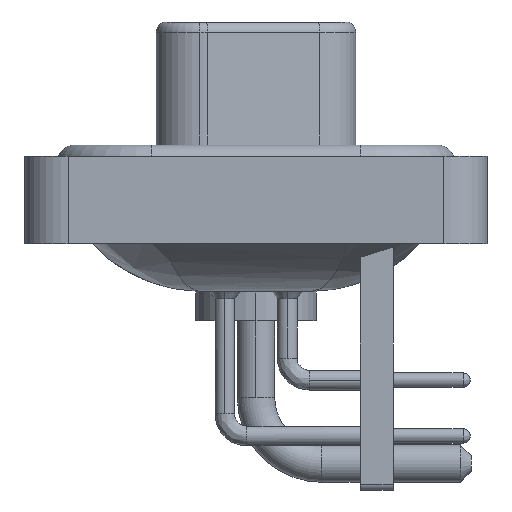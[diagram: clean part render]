
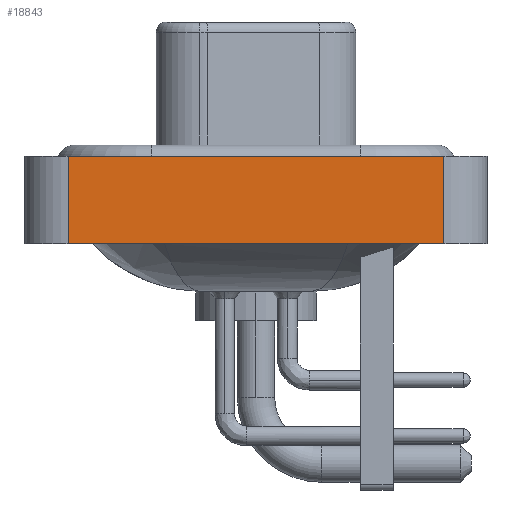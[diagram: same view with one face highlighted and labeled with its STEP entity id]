
A CAD part, left-side view. The second image highlights one B-rep face of the part: STEP entity #18843.
In plain terms, the highlighted planar face has unit normal (-1, 0, 0).
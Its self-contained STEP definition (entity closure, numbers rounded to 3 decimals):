
#630 = CARTESIAN_POINT ( 'NONE',  ( -7.25, -8.55, -3.6 ) ) ;
#1717 = EDGE_CURVE ( 'NONE', #21289, #21416, #18581, .T. ) ;
#2078 = EDGE_LOOP ( 'NONE', ( #3191, #15304, #12011, #8997 ) ) ;
#2207 = DIRECTION ( 'NONE',  ( 0., 0., 1. ) ) ;
#3191 = ORIENTED_EDGE ( 'NONE', *, *, #1717, .T. ) ;
#3697 = FACE_OUTER_BOUND ( 'NONE', #2078, .T. ) ;
#4210 = VECTOR ( 'NONE', #2207, 1000. ) ;
#4450 = DIRECTION ( 'NONE',  ( 0., -1., 0. ) ) ;
#5002 = DIRECTION ( 'NONE',  ( -1., 0., 0. ) ) ;
#5062 = LINE ( 'NONE', #12702, #16891 ) ;
#6217 = CARTESIAN_POINT ( 'NONE',  ( -7.25, -8.55, -3.6 ) ) ;
#8865 = LINE ( 'NONE', #19651, #16853 ) ;
#8997 = ORIENTED_EDGE ( 'NONE', *, *, #12492, .T. ) ;
#10084 = VERTEX_POINT ( 'NONE', #12901 ) ;
#10393 = CARTESIAN_POINT ( 'NONE',  ( -7.25, 8.55, -3.6 ) ) ;
#10760 = EDGE_CURVE ( 'NONE', #10084, #21416, #5062, .T. ) ;
#10972 = PLANE ( 'NONE',  #11722 ) ;
#11722 = AXIS2_PLACEMENT_3D ( 'NONE', #21378, #5002, #12288 ) ;
#12011 = ORIENTED_EDGE ( 'NONE', *, *, #14736, .F. ) ;
#12288 = DIRECTION ( 'NONE',  ( 0., 0., 1. ) ) ;
#12492 = EDGE_CURVE ( 'NONE', #16575, #21289, #17226, .T. ) ;
#12702 = CARTESIAN_POINT ( 'NONE',  ( -7.25, -8.55, 0.4 ) ) ;
#12901 = CARTESIAN_POINT ( 'NONE',  ( -7.25, 8.55, 0.4 ) ) ;
#14736 = EDGE_CURVE ( 'NONE', #16575, #10084, #8865, .T. ) ;
#15304 = ORIENTED_EDGE ( 'NONE', *, *, #10760, .F. ) ;
#15919 = CARTESIAN_POINT ( 'NONE',  ( -7.25, -8.55, -3.6 ) ) ;
#16049 = DIRECTION ( 'NONE',  ( 0., -1., 0. ) ) ;
#16575 = VERTEX_POINT ( 'NONE', #10393 ) ;
#16853 = VECTOR ( 'NONE', #23460, 1000. ) ;
#16891 = VECTOR ( 'NONE', #16049, 1000. ) ;
#17226 = LINE ( 'NONE', #630, #17584 ) ;
#17584 = VECTOR ( 'NONE', #4450, 1000. ) ;
#17590 = CARTESIAN_POINT ( 'NONE',  ( -7.25, -8.55, 0.4 ) ) ;
#18581 = LINE ( 'NONE', #6217, #4210 ) ;
#18843 = ADVANCED_FACE ( 'NONE', ( #3697 ), #10972, .T. ) ;
#19651 = CARTESIAN_POINT ( 'NONE',  ( -7.25, 8.55, -3.6 ) ) ;
#21289 = VERTEX_POINT ( 'NONE', #15919 ) ;
#21378 = CARTESIAN_POINT ( 'NONE',  ( -7.25, -8.55, -3.6 ) ) ;
#21416 = VERTEX_POINT ( 'NONE', #17590 ) ;
#23460 = DIRECTION ( 'NONE',  ( 0., 0., 1. ) ) ;
